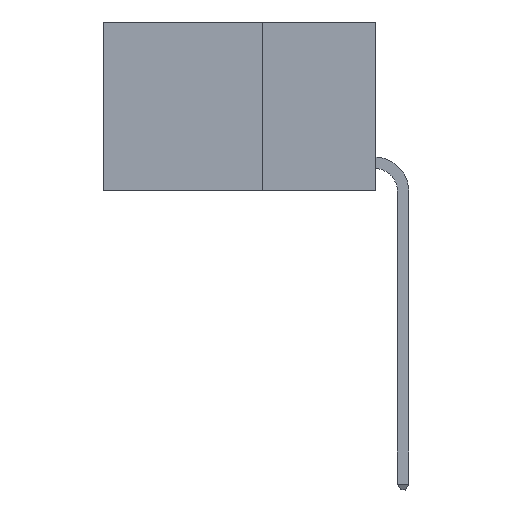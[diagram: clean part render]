
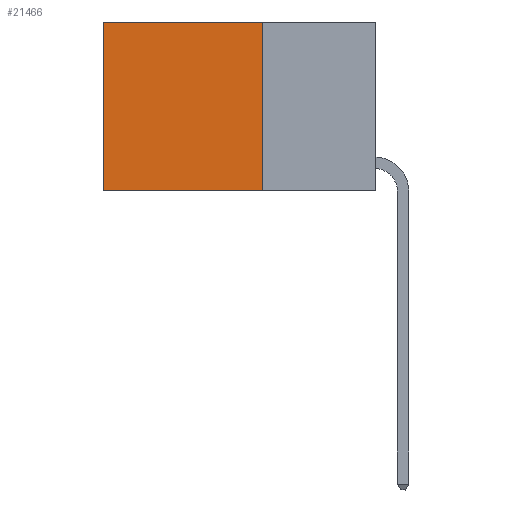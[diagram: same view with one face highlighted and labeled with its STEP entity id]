
A CAD part, left-side view. The second image highlights one B-rep face of the part: STEP entity #21466.
In plain terms, the highlighted planar face has unit normal (-1, 0, 0).
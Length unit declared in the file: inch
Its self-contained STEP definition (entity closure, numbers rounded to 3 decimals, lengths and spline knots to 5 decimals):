
#1632 = ORIENTED_EDGE ( 'NONE', *, *, #19790, .F. ) ;
#2134 = VERTEX_POINT ( 'NONE', #6880 ) ;
#2598 = DIRECTION ( 'NONE',  ( 0., 0., -1. ) ) ;
#3063 = DIRECTION ( 'NONE',  ( 1., 0., 0. ) ) ;
#3303 = EDGE_CURVE ( 'NONE', #2134, #14700, #10928, .T. ) ;
#4675 = ORIENTED_EDGE ( 'NONE', *, *, #7602, .F. ) ;
#4747 = CARTESIAN_POINT ( 'NONE',  ( 0.2625, 0.6, 0. ) ) ;
#4906 = CARTESIAN_POINT ( 'NONE',  ( 0.2625, 0.25, 0. ) ) ;
#5754 = EDGE_LOOP ( 'NONE', ( #11985, #1632, #4675, #7724 ) ) ;
#6313 = VECTOR ( 'NONE', #2598, 39.37008 ) ;
#6397 = EDGE_CURVE ( 'NONE', #14700, #20655, #20899, .T. ) ;
#6880 = CARTESIAN_POINT ( 'NONE',  ( 0.2625, 0.25, 0. ) ) ;
#7042 = CARTESIAN_POINT ( 'NONE',  ( 0.2625, 0.25, -0.37 ) ) ;
#7602 = EDGE_CURVE ( 'NONE', #2134, #20506, #13891, .T. ) ;
#7724 = ORIENTED_EDGE ( 'NONE', *, *, #3303, .T. ) ;
#10928 = LINE ( 'NONE', #4906, #17661 ) ;
#11061 = DIRECTION ( 'NONE',  ( 0., 1., 0. ) ) ;
#11985 = ORIENTED_EDGE ( 'NONE', *, *, #6397, .T. ) ;
#12030 = CARTESIAN_POINT ( 'NONE',  ( 0.2625, 0.25, -0.37 ) ) ;
#13253 = PLANE ( 'NONE',  #21155 ) ;
#13437 = CARTESIAN_POINT ( 'NONE',  ( 0.2625, 0.6, -0.37 ) ) ;
#13891 = LINE ( 'NONE', #20414, #14862 ) ;
#14700 = VERTEX_POINT ( 'NONE', #19817 ) ;
#14862 = VECTOR ( 'NONE', #20147, 39.37008 ) ;
#15494 = FACE_OUTER_BOUND ( 'NONE', #5754, .T. ) ;
#17635 = CARTESIAN_POINT ( 'NONE',  ( 0.2625, 0.25, 0. ) ) ;
#17661 = VECTOR ( 'NONE', #11061, 39.37008 ) ;
#19790 = EDGE_CURVE ( 'NONE', #20506, #20655, #26137, .T. ) ;
#19817 = CARTESIAN_POINT ( 'NONE',  ( 0.2625, 0.6, 0. ) ) ;
#20147 = DIRECTION ( 'NONE',  ( 0., 0., -1. ) ) ;
#20414 = CARTESIAN_POINT ( 'NONE',  ( 0.2625, 0.25, 0. ) ) ;
#20506 = VERTEX_POINT ( 'NONE', #7042 ) ;
#20655 = VERTEX_POINT ( 'NONE', #13437 ) ;
#20899 = LINE ( 'NONE', #4747, #6313 ) ;
#21155 = AXIS2_PLACEMENT_3D ( 'NONE', #17635, #3063, #26245 ) ;
#21466 = ADVANCED_FACE ( 'NONE', ( #15494 ), #13253, .F. ) ;
#24023 = DIRECTION ( 'NONE',  ( 0., 1., 0. ) ) ;
#26136 = VECTOR ( 'NONE', #24023, 39.37008 ) ;
#26137 = LINE ( 'NONE', #12030, #26136 ) ;
#26245 = DIRECTION ( 'NONE',  ( 0., 0., -1. ) ) ;
